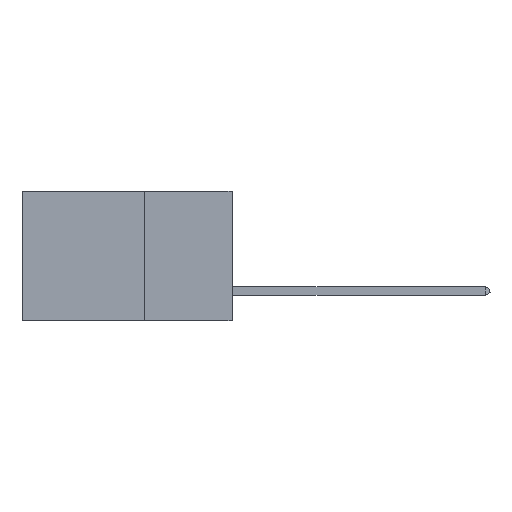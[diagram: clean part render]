
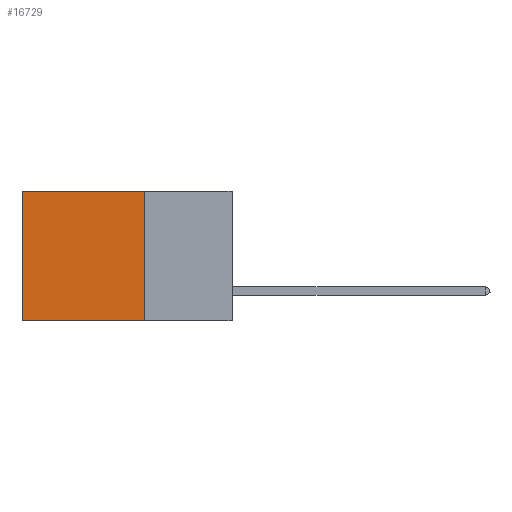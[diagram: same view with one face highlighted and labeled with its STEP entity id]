
A CAD part, left-side view. The second image highlights one B-rep face of the part: STEP entity #16729.
In plain terms, the highlighted planar face has unit normal (-1, 0, 0).
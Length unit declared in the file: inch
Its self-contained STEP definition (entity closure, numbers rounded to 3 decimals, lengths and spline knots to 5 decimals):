
#2513 = ORIENTED_EDGE ( 'NONE', *, *, #14196, .F. ) ;
#2518 = CARTESIAN_POINT ( 'NONE',  ( 0.2875, 0.25, 0. ) ) ;
#2898 = VECTOR ( 'NONE', #5631, 39.37008 ) ;
#3071 = ORIENTED_EDGE ( 'NONE', *, *, #21225, .F. ) ;
#5004 = DIRECTION ( 'NONE',  ( 0., 1., 0. ) ) ;
#5631 = DIRECTION ( 'NONE',  ( 0., 0., -1. ) ) ;
#5653 = VERTEX_POINT ( 'NONE', #25121 ) ;
#6947 = CARTESIAN_POINT ( 'NONE',  ( 0.2875, 0.6, 0. ) ) ;
#9118 = CARTESIAN_POINT ( 'NONE',  ( 0.2875, 0.25, -0.37 ) ) ;
#9639 = VERTEX_POINT ( 'NONE', #13658 ) ;
#10664 = VECTOR ( 'NONE', #5004, 39.37008 ) ;
#11657 = PLANE ( 'NONE',  #16995 ) ;
#13243 = DIRECTION ( 'NONE',  ( 0., 1., 0. ) ) ;
#13658 = CARTESIAN_POINT ( 'NONE',  ( 0.2875, 0.25, 0. ) ) ;
#14131 = EDGE_LOOP ( 'NONE', ( #23725, #3071, #2513, #21688 ) ) ;
#14196 = EDGE_CURVE ( 'NONE', #9639, #30174, #16362, .T. ) ;
#14808 = LINE ( 'NONE', #2518, #10664 ) ;
#16362 = LINE ( 'NONE', #28694, #28576 ) ;
#16454 = CARTESIAN_POINT ( 'NONE',  ( 0.2875, 0.25, 0. ) ) ;
#16729 = ADVANCED_FACE ( 'NONE', ( #18936 ), #11657, .F. ) ;
#16995 = AXIS2_PLACEMENT_3D ( 'NONE', #16454, #28733, #21393 ) ;
#17793 = EDGE_CURVE ( 'NONE', #25998, #5653, #31180, .T. ) ;
#18936 = FACE_OUTER_BOUND ( 'NONE', #14131, .T. ) ;
#20219 = CARTESIAN_POINT ( 'NONE',  ( 0.2875, 0.6, 0. ) ) ;
#21225 = EDGE_CURVE ( 'NONE', #30174, #5653, #22138, .T. ) ;
#21393 = DIRECTION ( 'NONE',  ( 0., 0., -1. ) ) ;
#21688 = ORIENTED_EDGE ( 'NONE', *, *, #29548, .T. ) ;
#22138 = LINE ( 'NONE', #9118, #26723 ) ;
#23443 = CARTESIAN_POINT ( 'NONE',  ( 0.2875, 0.25, -0.37 ) ) ;
#23725 = ORIENTED_EDGE ( 'NONE', *, *, #17793, .T. ) ;
#25121 = CARTESIAN_POINT ( 'NONE',  ( 0.2875, 0.6, -0.37 ) ) ;
#25998 = VERTEX_POINT ( 'NONE', #6947 ) ;
#26723 = VECTOR ( 'NONE', #13243, 39.37008 ) ;
#28576 = VECTOR ( 'NONE', #30840, 39.37008 ) ;
#28694 = CARTESIAN_POINT ( 'NONE',  ( 0.2875, 0.25, 0. ) ) ;
#28733 = DIRECTION ( 'NONE',  ( 1., 0., 0. ) ) ;
#29548 = EDGE_CURVE ( 'NONE', #9639, #25998, #14808, .T. ) ;
#30174 = VERTEX_POINT ( 'NONE', #23443 ) ;
#30840 = DIRECTION ( 'NONE',  ( 0., 0., -1. ) ) ;
#31180 = LINE ( 'NONE', #20219, #2898 ) ;
